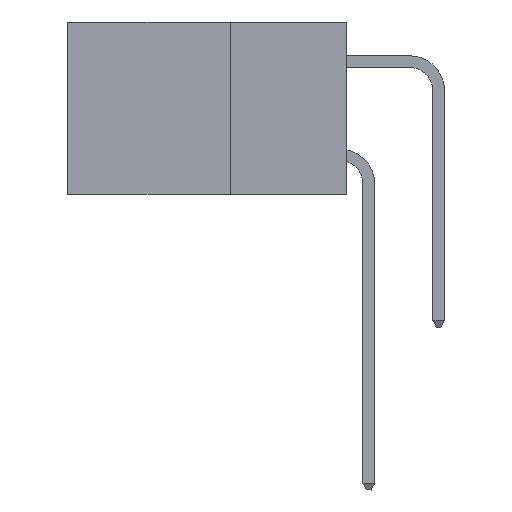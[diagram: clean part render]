
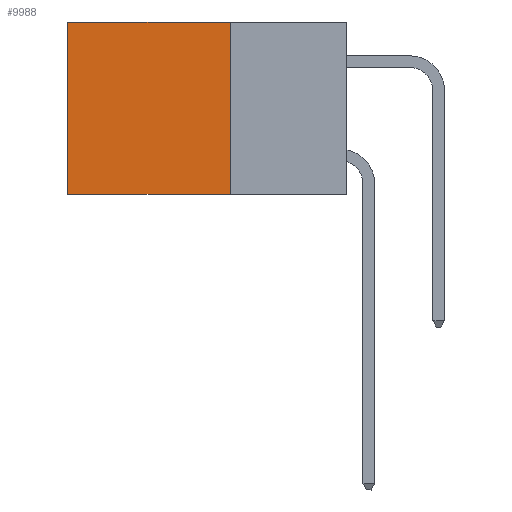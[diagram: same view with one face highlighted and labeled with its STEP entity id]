
A CAD part, left-side view. The second image highlights one B-rep face of the part: STEP entity #9988.
In plain terms, the highlighted planar face has unit normal (-1, 0, 0).
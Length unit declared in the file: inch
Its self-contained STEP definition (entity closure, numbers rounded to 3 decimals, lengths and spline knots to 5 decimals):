
#286 = LINE ( 'NONE', #10019, #13407 ) ;
#391 = DIRECTION ( 'NONE',  ( 0., 0., -1. ) ) ;
#521 = EDGE_CURVE ( 'NONE', #19444, #10534, #18004, .T. ) ;
#690 = DIRECTION ( 'NONE',  ( 0., 1., 0. ) ) ;
#1924 = ORIENTED_EDGE ( 'NONE', *, *, #19303, .F. ) ;
#3778 = VECTOR ( 'NONE', #690, 39.37008 ) ;
#4237 = PLANE ( 'NONE',  #9167 ) ;
#4321 = LINE ( 'NONE', #7681, #3778 ) ;
#4720 = ORIENTED_EDGE ( 'NONE', *, *, #17298, .F. ) ;
#4844 = CARTESIAN_POINT ( 'NONE',  ( 0.2875, 0.6, -0.37 ) ) ;
#5082 = EDGE_LOOP ( 'NONE', ( #11336, #1924, #4720, #5466 ) ) ;
#5466 = ORIENTED_EDGE ( 'NONE', *, *, #13517, .T. ) ;
#5522 = LINE ( 'NONE', #6937, #17487 ) ;
#6937 = CARTESIAN_POINT ( 'NONE',  ( 0.2875, 0.25, 0. ) ) ;
#7681 = CARTESIAN_POINT ( 'NONE',  ( 0.2875, 0.25, -0.37 ) ) ;
#8765 = CARTESIAN_POINT ( 'NONE',  ( 0.2875, 0.25, 0. ) ) ;
#9167 = AXIS2_PLACEMENT_3D ( 'NONE', #10972, #17470, #17579 ) ;
#9446 = CARTESIAN_POINT ( 'NONE',  ( 0.2875, 0.6, 0. ) ) ;
#9988 = ADVANCED_FACE ( 'NONE', ( #12590 ), #4237, .F. ) ;
#10019 = CARTESIAN_POINT ( 'NONE',  ( 0.2875, 0.25, 0. ) ) ;
#10534 = VERTEX_POINT ( 'NONE', #4844 ) ;
#10972 = CARTESIAN_POINT ( 'NONE',  ( 0.2875, 0.25, 0. ) ) ;
#11336 = ORIENTED_EDGE ( 'NONE', *, *, #521, .T. ) ;
#12226 = VERTEX_POINT ( 'NONE', #8765 ) ;
#12590 = FACE_OUTER_BOUND ( 'NONE', #5082, .T. ) ;
#13407 = VECTOR ( 'NONE', #391, 39.37008 ) ;
#13517 = EDGE_CURVE ( 'NONE', #12226, #19444, #5522, .T. ) ;
#13555 = DIRECTION ( 'NONE',  ( 0., 1., 0. ) ) ;
#14544 = DIRECTION ( 'NONE',  ( 0., 0., -1. ) ) ;
#15483 = VERTEX_POINT ( 'NONE', #17629 ) ;
#16817 = VECTOR ( 'NONE', #14544, 39.37008 ) ;
#17298 = EDGE_CURVE ( 'NONE', #12226, #15483, #286, .T. ) ;
#17470 = DIRECTION ( 'NONE',  ( 1., 0., 0. ) ) ;
#17487 = VECTOR ( 'NONE', #13555, 39.37008 ) ;
#17579 = DIRECTION ( 'NONE',  ( 0., 0., -1. ) ) ;
#17629 = CARTESIAN_POINT ( 'NONE',  ( 0.2875, 0.25, -0.37 ) ) ;
#18004 = LINE ( 'NONE', #9446, #16817 ) ;
#18087 = CARTESIAN_POINT ( 'NONE',  ( 0.2875, 0.6, 0. ) ) ;
#19303 = EDGE_CURVE ( 'NONE', #15483, #10534, #4321, .T. ) ;
#19444 = VERTEX_POINT ( 'NONE', #18087 ) ;
